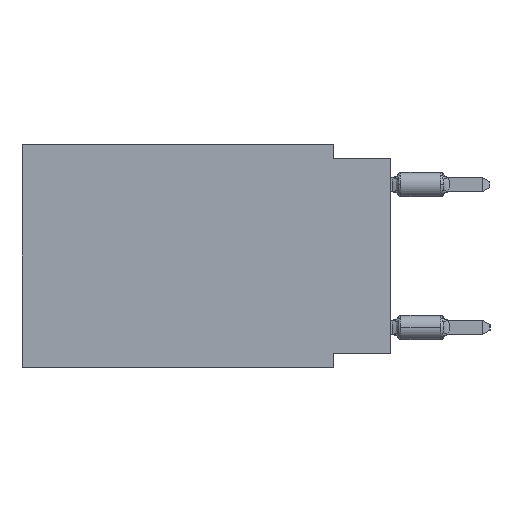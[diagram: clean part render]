
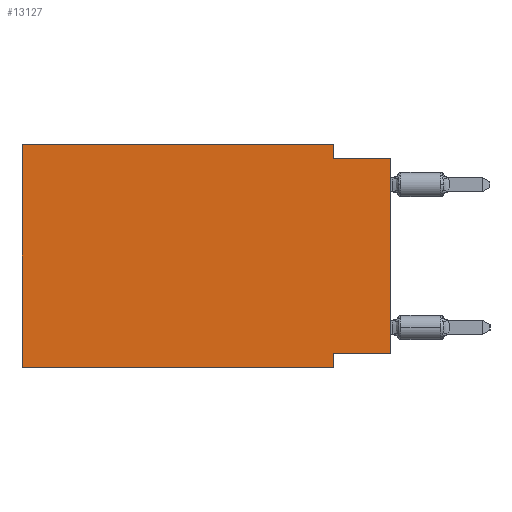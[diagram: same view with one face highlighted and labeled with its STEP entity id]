
A CAD part, left-side view. The second image highlights one B-rep face of the part: STEP entity #13127.
In plain terms, the highlighted planar face has unit normal (-1, 0, 0).
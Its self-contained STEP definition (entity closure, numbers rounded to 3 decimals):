
#127 = VERTEX_POINT ( 'NONE', #8848 ) ;
#1075 = CARTESIAN_POINT ( 'NONE',  ( 0., 2.54, -9.271 ) ) ;
#2304 = VECTOR ( 'NONE', #26539, 1000. ) ;
#2540 = ORIENTED_EDGE ( 'NONE', *, *, #18585, .F. ) ;
#2956 = CARTESIAN_POINT ( 'NONE',  ( 0., 2.54, 0. ) ) ;
#3276 = CARTESIAN_POINT ( 'NONE',  ( 0., 16.383, 0. ) ) ;
#3295 = CARTESIAN_POINT ( 'NONE',  ( 0., 0., -0.635 ) ) ;
#3780 = LINE ( 'NONE', #28721, #39289 ) ;
#4741 = EDGE_CURVE ( 'NONE', #14268, #15013, #16103, .T. ) ;
#6250 = LINE ( 'NONE', #46930, #6352 ) ;
#6335 = CARTESIAN_POINT ( 'NONE',  ( 0., 2.54, -9.906 ) ) ;
#6352 = VECTOR ( 'NONE', #10322, 1000. ) ;
#6522 = VERTEX_POINT ( 'NONE', #20575 ) ;
#8848 = CARTESIAN_POINT ( 'NONE',  ( 0., 16.383, -9.906 ) ) ;
#10144 = CARTESIAN_POINT ( 'NONE',  ( 0., 0., -9.271 ) ) ;
#10322 = DIRECTION ( 'NONE',  ( 0., -1., 0. ) ) ;
#11652 = CARTESIAN_POINT ( 'NONE',  ( 0., 16.383, 0. ) ) ;
#11839 = LINE ( 'NONE', #36782, #32148 ) ;
#13127 = ADVANCED_FACE ( 'NONE', ( #44075 ), #36445, .F. ) ;
#14070 = CARTESIAN_POINT ( 'NONE',  ( 0., 2.54, 0. ) ) ;
#14264 = EDGE_LOOP ( 'NONE', ( #49015, #39934, #2540, #42544, #31780, #40683, #20867, #18597 ) ) ;
#14268 = VERTEX_POINT ( 'NONE', #10144 ) ;
#14867 = EDGE_CURVE ( 'NONE', #14268, #21744, #32810, .T. ) ;
#15013 = VERTEX_POINT ( 'NONE', #1075 ) ;
#16103 = LINE ( 'NONE', #24791, #50993 ) ;
#16383 = DIRECTION ( 'NONE',  ( 0., 1., 0. ) ) ;
#17749 = EDGE_CURVE ( 'NONE', #15013, #6522, #35608, .T. ) ;
#18585 = EDGE_CURVE ( 'NONE', #27267, #20164, #51230, .T. ) ;
#18597 = ORIENTED_EDGE ( 'NONE', *, *, #4741, .F. ) ;
#20164 = VERTEX_POINT ( 'NONE', #22689 ) ;
#20575 = CARTESIAN_POINT ( 'NONE',  ( 0., 2.54, -9.906 ) ) ;
#20867 = ORIENTED_EDGE ( 'NONE', *, *, #17749, .F. ) ;
#21744 = VERTEX_POINT ( 'NONE', #3295 ) ;
#22059 = EDGE_CURVE ( 'NONE', #20164, #21744, #6250, .T. ) ;
#22109 = EDGE_CURVE ( 'NONE', #127, #6522, #3780, .T. ) ;
#22689 = CARTESIAN_POINT ( 'NONE',  ( 0., 2.54, -0.635 ) ) ;
#23353 = VERTEX_POINT ( 'NONE', #11652 ) ;
#24696 = CARTESIAN_POINT ( 'NONE',  ( 0., 0., 0. ) ) ;
#24791 = CARTESIAN_POINT ( 'NONE',  ( 0., 0., -9.271 ) ) ;
#25508 = AXIS2_PLACEMENT_3D ( 'NONE', #28303, #28048, #32373 ) ;
#26539 = DIRECTION ( 'NONE',  ( 0., 0., -1. ) ) ;
#27053 = EDGE_CURVE ( 'NONE', #23353, #27267, #44516, .T. ) ;
#27267 = VERTEX_POINT ( 'NONE', #2956 ) ;
#28048 = DIRECTION ( 'NONE',  ( 1., 0., 0. ) ) ;
#28303 = CARTESIAN_POINT ( 'NONE',  ( 0., 16.383, 0. ) ) ;
#28721 = CARTESIAN_POINT ( 'NONE',  ( 0., 16.383, -9.906 ) ) ;
#30306 = VECTOR ( 'NONE', #42027, 1000. ) ;
#31638 = EDGE_CURVE ( 'NONE', #127, #23353, #11839, .T. ) ;
#31693 = VECTOR ( 'NONE', #43759, 1000. ) ;
#31780 = ORIENTED_EDGE ( 'NONE', *, *, #31638, .F. ) ;
#32148 = VECTOR ( 'NONE', #53319, 1000. ) ;
#32289 = DIRECTION ( 'NONE',  ( 0., -1., 0. ) ) ;
#32373 = DIRECTION ( 'NONE',  ( 0., 0., -1. ) ) ;
#32810 = LINE ( 'NONE', #24696, #30306 ) ;
#35608 = LINE ( 'NONE', #6335, #31693 ) ;
#36445 = PLANE ( 'NONE',  #25508 ) ;
#36782 = CARTESIAN_POINT ( 'NONE',  ( 0., 16.383, 0. ) ) ;
#39289 = VECTOR ( 'NONE', #53386, 1000. ) ;
#39934 = ORIENTED_EDGE ( 'NONE', *, *, #22059, .F. ) ;
#40683 = ORIENTED_EDGE ( 'NONE', *, *, #22109, .T. ) ;
#42027 = DIRECTION ( 'NONE',  ( 0., 0., 1. ) ) ;
#42544 = ORIENTED_EDGE ( 'NONE', *, *, #27053, .F. ) ;
#43759 = DIRECTION ( 'NONE',  ( 0., 0., -1. ) ) ;
#44075 = FACE_OUTER_BOUND ( 'NONE', #14264, .T. ) ;
#44516 = LINE ( 'NONE', #3276, #48461 ) ;
#46930 = CARTESIAN_POINT ( 'NONE',  ( 0., 0., -0.635 ) ) ;
#48461 = VECTOR ( 'NONE', #32289, 1000. ) ;
#49015 = ORIENTED_EDGE ( 'NONE', *, *, #14867, .T. ) ;
#50993 = VECTOR ( 'NONE', #16383, 1000. ) ;
#51230 = LINE ( 'NONE', #14070, #2304 ) ;
#53319 = DIRECTION ( 'NONE',  ( 0., 0., 1. ) ) ;
#53386 = DIRECTION ( 'NONE',  ( 0., -1., 0. ) ) ;
